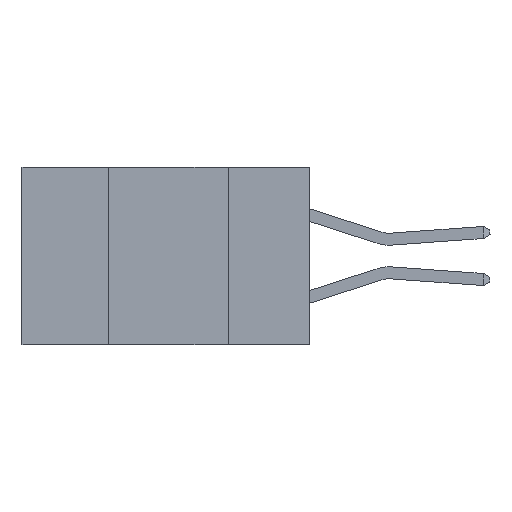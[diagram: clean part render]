
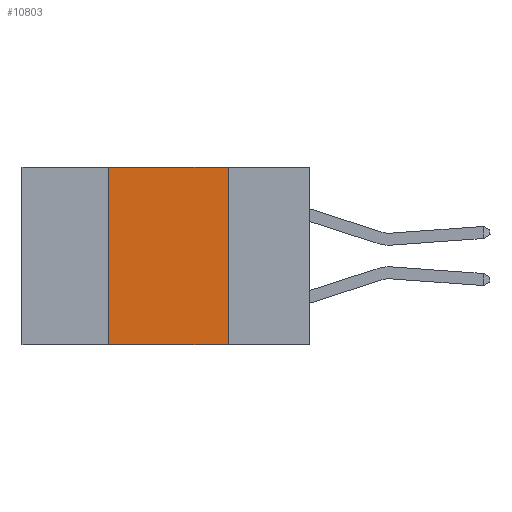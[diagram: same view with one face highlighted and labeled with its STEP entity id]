
A CAD part, left-side view. The second image highlights one B-rep face of the part: STEP entity #10803.
In plain terms, the highlighted planar face has unit normal (-1, 0, 0).
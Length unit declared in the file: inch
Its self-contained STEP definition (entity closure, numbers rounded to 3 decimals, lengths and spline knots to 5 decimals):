
#10 = FACE_OUTER_BOUND ( 'NONE', #8459, .T. ) ;
#697 = VERTEX_POINT ( 'NONE', #9920 ) ;
#911 = ORIENTED_EDGE ( 'NONE', *, *, #10006, .F. ) ;
#1832 = LINE ( 'NONE', #1962, #7893 ) ;
#1962 = CARTESIAN_POINT ( 'NONE',  ( 0., 0.42, -0.37 ) ) ;
#2199 = AXIS2_PLACEMENT_3D ( 'NONE', #12879, #4483, #13094 ) ;
#2716 = CARTESIAN_POINT ( 'NONE',  ( 0., 0.6, -0.37 ) ) ;
#2809 = LINE ( 'NONE', #12506, #10786 ) ;
#3573 = VECTOR ( 'NONE', #11640, 39.37008 ) ;
#3873 = VERTEX_POINT ( 'NONE', #6807 ) ;
#4483 = DIRECTION ( 'NONE',  ( 1., 0., 0. ) ) ;
#6338 = EDGE_CURVE ( 'NONE', #3873, #8780, #2809, .T. ) ;
#6495 = ORIENTED_EDGE ( 'NONE', *, *, #13222, .T. ) ;
#6511 = VERTEX_POINT ( 'NONE', #10570 ) ;
#6807 = CARTESIAN_POINT ( 'NONE',  ( 0., 0.42, 0. ) ) ;
#7093 = ORIENTED_EDGE ( 'NONE', *, *, #12005, .F. ) ;
#7602 = ORIENTED_EDGE ( 'NONE', *, *, #6338, .F. ) ;
#7893 = VECTOR ( 'NONE', #10561, 39.37008 ) ;
#7969 = LINE ( 'NONE', #2716, #9989 ) ;
#8308 = CARTESIAN_POINT ( 'NONE',  ( 0., 0.17, -0.37 ) ) ;
#8459 = EDGE_LOOP ( 'NONE', ( #911, #7602, #7093, #6495 ) ) ;
#8590 = PLANE ( 'NONE',  #2199 ) ;
#8780 = VERTEX_POINT ( 'NONE', #9013 ) ;
#9013 = CARTESIAN_POINT ( 'NONE',  ( 0., 0.17, 0. ) ) ;
#9920 = CARTESIAN_POINT ( 'NONE',  ( 0., 0.42, -0.37 ) ) ;
#9989 = VECTOR ( 'NONE', #11328, 39.37008 ) ;
#10006 = EDGE_CURVE ( 'NONE', #8780, #6511, #10581, .T. ) ;
#10561 = DIRECTION ( 'NONE',  ( 0., 0., 1. ) ) ;
#10570 = CARTESIAN_POINT ( 'NONE',  ( 0., 0.17, -0.37 ) ) ;
#10581 = LINE ( 'NONE', #8308, #3573 ) ;
#10786 = VECTOR ( 'NONE', #11360, 39.37008 ) ;
#10803 = ADVANCED_FACE ( 'NONE', ( #10 ), #8590, .F. ) ;
#11328 = DIRECTION ( 'NONE',  ( 0., -1., 0. ) ) ;
#11360 = DIRECTION ( 'NONE',  ( 0., -1., 0. ) ) ;
#11640 = DIRECTION ( 'NONE',  ( 0., 0., -1. ) ) ;
#12005 = EDGE_CURVE ( 'NONE', #697, #3873, #1832, .T. ) ;
#12506 = CARTESIAN_POINT ( 'NONE',  ( 0., 0.6, 0. ) ) ;
#12879 = CARTESIAN_POINT ( 'NONE',  ( 0., 0.6, 0. ) ) ;
#13094 = DIRECTION ( 'NONE',  ( 0., 0., -1. ) ) ;
#13222 = EDGE_CURVE ( 'NONE', #697, #6511, #7969, .T. ) ;
